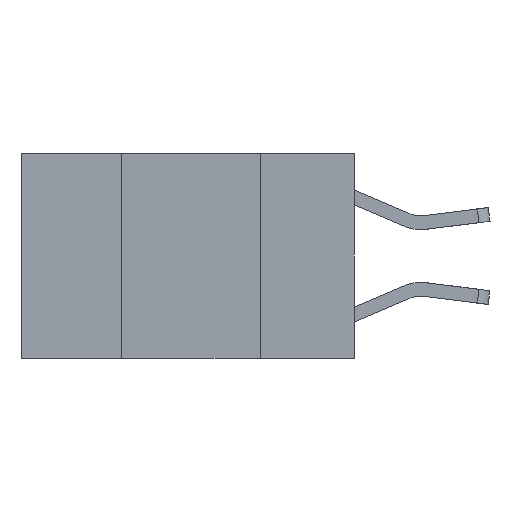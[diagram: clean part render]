
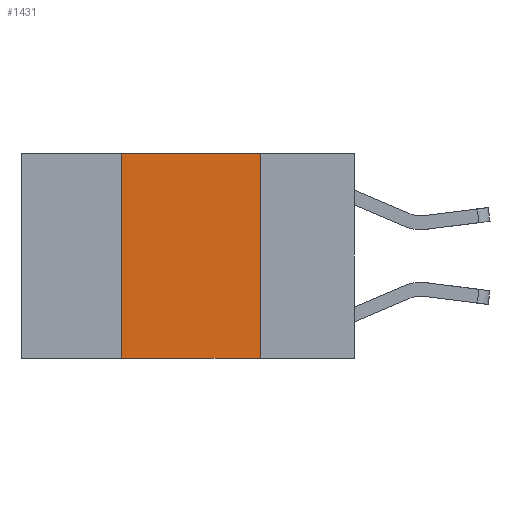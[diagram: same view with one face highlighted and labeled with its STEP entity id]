
A CAD part, left-side view. The second image highlights one B-rep face of the part: STEP entity #1431.
In plain terms, the highlighted planar face has unit normal (-1, 0, 0).
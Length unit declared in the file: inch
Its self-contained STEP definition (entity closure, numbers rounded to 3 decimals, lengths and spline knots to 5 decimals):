
#74 = ORIENTED_EDGE ( 'NONE', *, *, #9089, .F. ) ;
#156 = CARTESIAN_POINT ( 'NONE',  ( 0., 0.42, 0. ) ) ;
#442 = LINE ( 'NONE', #1015, #4514 ) ;
#730 = DIRECTION ( 'NONE',  ( 0., 0., -1. ) ) ;
#734 = CARTESIAN_POINT ( 'NONE',  ( 0., 0.6, 0. ) ) ;
#959 = CARTESIAN_POINT ( 'NONE',  ( 0., 0.6, 0. ) ) ;
#1015 = CARTESIAN_POINT ( 'NONE',  ( 0., 0.17, 0. ) ) ;
#1025 = VECTOR ( 'NONE', #10499, 39.37008 ) ;
#1389 = ORIENTED_EDGE ( 'NONE', *, *, #5860, .F. ) ;
#1431 = ADVANCED_FACE ( 'NONE', ( #4581 ), #9978, .F. ) ;
#2262 = LINE ( 'NONE', #156, #8509 ) ;
#2397 = EDGE_LOOP ( 'NONE', ( #10582, #1389, #74, #4957 ) ) ;
#2812 = CARTESIAN_POINT ( 'NONE',  ( 0., 0.6, -0.37 ) ) ;
#3262 = AXIS2_PLACEMENT_3D ( 'NONE', #959, #6151, #730 ) ;
#3674 = DIRECTION ( 'NONE',  ( 0., -1., 0. ) ) ;
#4264 = VECTOR ( 'NONE', #3674, 39.37008 ) ;
#4514 = VECTOR ( 'NONE', #6893, 39.37008 ) ;
#4581 = FACE_OUTER_BOUND ( 'NONE', #2397, .T. ) ;
#4784 = VERTEX_POINT ( 'NONE', #8414 ) ;
#4957 = ORIENTED_EDGE ( 'NONE', *, *, #9096, .T. ) ;
#5185 = CARTESIAN_POINT ( 'NONE',  ( 0., 0.42, 0. ) ) ;
#5860 = EDGE_CURVE ( 'NONE', #9866, #6462, #10221, .T. ) ;
#6134 = DIRECTION ( 'NONE',  ( 0., 0., 1. ) ) ;
#6151 = DIRECTION ( 'NONE',  ( 1., 0., 0. ) ) ;
#6462 = VERTEX_POINT ( 'NONE', #7149 ) ;
#6614 = VERTEX_POINT ( 'NONE', #9008 ) ;
#6692 = LINE ( 'NONE', #2812, #4264 ) ;
#6893 = DIRECTION ( 'NONE',  ( 0., 0., -1. ) ) ;
#7149 = CARTESIAN_POINT ( 'NONE',  ( 0., 0.17, 0. ) ) ;
#8414 = CARTESIAN_POINT ( 'NONE',  ( 0., 0.17, -0.37 ) ) ;
#8509 = VECTOR ( 'NONE', #6134, 39.37008 ) ;
#9008 = CARTESIAN_POINT ( 'NONE',  ( 0., 0.42, -0.37 ) ) ;
#9053 = EDGE_CURVE ( 'NONE', #6462, #4784, #442, .T. ) ;
#9089 = EDGE_CURVE ( 'NONE', #6614, #9866, #2262, .T. ) ;
#9096 = EDGE_CURVE ( 'NONE', #6614, #4784, #6692, .T. ) ;
#9866 = VERTEX_POINT ( 'NONE', #5185 ) ;
#9978 = PLANE ( 'NONE',  #3262 ) ;
#10221 = LINE ( 'NONE', #734, #1025 ) ;
#10499 = DIRECTION ( 'NONE',  ( 0., -1., 0. ) ) ;
#10582 = ORIENTED_EDGE ( 'NONE', *, *, #9053, .F. ) ;
